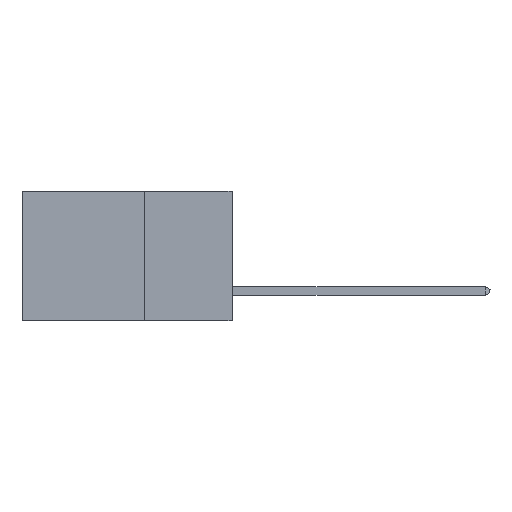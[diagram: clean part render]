
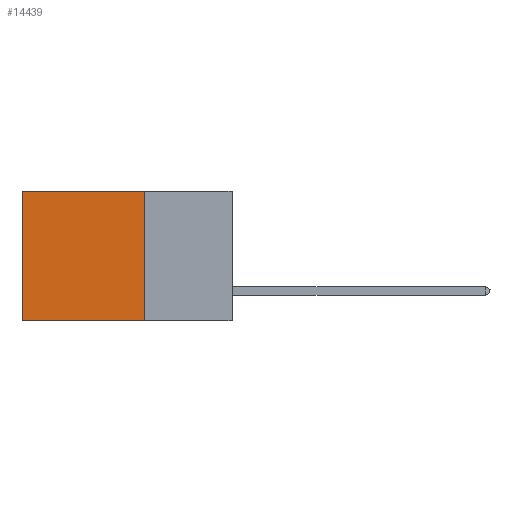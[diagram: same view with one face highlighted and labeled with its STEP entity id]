
A CAD part, left-side view. The second image highlights one B-rep face of the part: STEP entity #14439.
In plain terms, the highlighted planar face has unit normal (-1, 0, 0).
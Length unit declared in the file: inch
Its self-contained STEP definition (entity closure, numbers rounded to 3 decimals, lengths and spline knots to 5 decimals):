
#399 = DIRECTION ( 'NONE',  ( 0., 0., -1. ) ) ;
#876 = ORIENTED_EDGE ( 'NONE', *, *, #17279, .F. ) ;
#1591 = CARTESIAN_POINT ( 'NONE',  ( 0.2875, 0.25, 0. ) ) ;
#1613 = AXIS2_PLACEMENT_3D ( 'NONE', #8739, #2078, #4703 ) ;
#1614 = LINE ( 'NONE', #16334, #11508 ) ;
#2078 = DIRECTION ( 'NONE',  ( 1., 0., 0. ) ) ;
#3239 = CARTESIAN_POINT ( 'NONE',  ( 0.2875, 0.25, 0. ) ) ;
#3318 = PLANE ( 'NONE',  #1613 ) ;
#3945 = CARTESIAN_POINT ( 'NONE',  ( 0.2875, 0.6, 0. ) ) ;
#4447 = VERTEX_POINT ( 'NONE', #6644 ) ;
#4630 = VERTEX_POINT ( 'NONE', #1591 ) ;
#4666 = CARTESIAN_POINT ( 'NONE',  ( 0.2875, 0.6, 0. ) ) ;
#4703 = DIRECTION ( 'NONE',  ( 0., 0., -1. ) ) ;
#5572 = EDGE_CURVE ( 'NONE', #4630, #14026, #9607, .T. ) ;
#5865 = CARTESIAN_POINT ( 'NONE',  ( 0.2875, 0.25, 0. ) ) ;
#6228 = LINE ( 'NONE', #4666, #9122 ) ;
#6644 = CARTESIAN_POINT ( 'NONE',  ( 0.2875, 0.6, -0.37 ) ) ;
#6645 = EDGE_CURVE ( 'NONE', #14026, #4447, #6228, .T. ) ;
#7353 = DIRECTION ( 'NONE',  ( 0., 0., -1. ) ) ;
#7814 = ORIENTED_EDGE ( 'NONE', *, *, #6645, .T. ) ;
#8335 = DIRECTION ( 'NONE',  ( 0., 1., 0. ) ) ;
#8739 = CARTESIAN_POINT ( 'NONE',  ( 0.2875, 0.25, 0. ) ) ;
#9122 = VECTOR ( 'NONE', #7353, 39.37008 ) ;
#9607 = LINE ( 'NONE', #5865, #16104 ) ;
#9960 = VERTEX_POINT ( 'NONE', #11865 ) ;
#10441 = LINE ( 'NONE', #3239, #17146 ) ;
#10915 = ORIENTED_EDGE ( 'NONE', *, *, #5572, .T. ) ;
#11508 = VECTOR ( 'NONE', #8335, 39.37008 ) ;
#11865 = CARTESIAN_POINT ( 'NONE',  ( 0.2875, 0.25, -0.37 ) ) ;
#12200 = EDGE_LOOP ( 'NONE', ( #7814, #13874, #876, #10915 ) ) ;
#13874 = ORIENTED_EDGE ( 'NONE', *, *, #16347, .F. ) ;
#14026 = VERTEX_POINT ( 'NONE', #3945 ) ;
#14028 = DIRECTION ( 'NONE',  ( 0., 1., 0. ) ) ;
#14439 = ADVANCED_FACE ( 'NONE', ( #16523 ), #3318, .F. ) ;
#16104 = VECTOR ( 'NONE', #14028, 39.37008 ) ;
#16334 = CARTESIAN_POINT ( 'NONE',  ( 0.2875, 0.25, -0.37 ) ) ;
#16347 = EDGE_CURVE ( 'NONE', #9960, #4447, #1614, .T. ) ;
#16523 = FACE_OUTER_BOUND ( 'NONE', #12200, .T. ) ;
#17146 = VECTOR ( 'NONE', #399, 39.37008 ) ;
#17279 = EDGE_CURVE ( 'NONE', #4630, #9960, #10441, .T. ) ;
